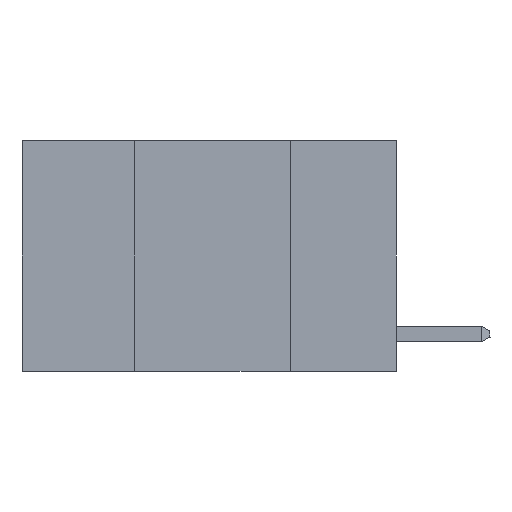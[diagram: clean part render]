
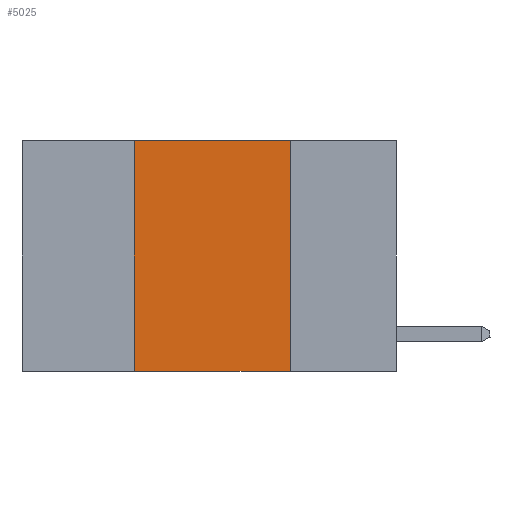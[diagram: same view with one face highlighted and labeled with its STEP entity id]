
A CAD part, left-side view. The second image highlights one B-rep face of the part: STEP entity #5025.
In plain terms, the highlighted planar face has unit normal (-1, 0, 0).
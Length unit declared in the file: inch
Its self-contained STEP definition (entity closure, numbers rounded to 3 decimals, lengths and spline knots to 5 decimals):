
#17 = LINE ( 'NONE', #2083, #7392 ) ;
#215 = CARTESIAN_POINT ( 'NONE',  ( 0., 0.42, 0. ) ) ;
#430 = CARTESIAN_POINT ( 'NONE',  ( 0., 0.6, 0. ) ) ;
#497 = EDGE_CURVE ( 'NONE', #7032, #1361, #4445, .T. ) ;
#557 = VERTEX_POINT ( 'NONE', #215 ) ;
#1181 = ORIENTED_EDGE ( 'NONE', *, *, #2107, .T. ) ;
#1361 = VERTEX_POINT ( 'NONE', #7373 ) ;
#1460 = CARTESIAN_POINT ( 'NONE',  ( 0., 0.17, 0. ) ) ;
#1609 = EDGE_CURVE ( 'NONE', #4319, #557, #2614, .T. ) ;
#1966 = DIRECTION ( 'NONE',  ( 0., 0., -1. ) ) ;
#1973 = DIRECTION ( 'NONE',  ( 0., -1., 0. ) ) ;
#2083 = CARTESIAN_POINT ( 'NONE',  ( 0., 0.6, -0.37 ) ) ;
#2107 = EDGE_CURVE ( 'NONE', #4319, #1361, #17, .T. ) ;
#2372 = ORIENTED_EDGE ( 'NONE', *, *, #1609, .F. ) ;
#2577 = PLANE ( 'NONE',  #3948 ) ;
#2614 = LINE ( 'NONE', #8236, #7128 ) ;
#3089 = ORIENTED_EDGE ( 'NONE', *, *, #4237, .F. ) ;
#3349 = CARTESIAN_POINT ( 'NONE',  ( 0., 0.6, 0. ) ) ;
#3557 = VECTOR ( 'NONE', #1973, 39.37008 ) ;
#3948 = AXIS2_PLACEMENT_3D ( 'NONE', #3349, #4789, #1966 ) ;
#4237 = EDGE_CURVE ( 'NONE', #557, #7032, #5991, .T. ) ;
#4319 = VERTEX_POINT ( 'NONE', #6318 ) ;
#4445 = LINE ( 'NONE', #8142, #8303 ) ;
#4789 = DIRECTION ( 'NONE',  ( 1., 0., 0. ) ) ;
#5025 = ADVANCED_FACE ( 'NONE', ( #6854 ), #2577, .F. ) ;
#5581 = ORIENTED_EDGE ( 'NONE', *, *, #497, .F. ) ;
#5991 = LINE ( 'NONE', #430, #3557 ) ;
#6318 = CARTESIAN_POINT ( 'NONE',  ( 0., 0.42, -0.37 ) ) ;
#6854 = FACE_OUTER_BOUND ( 'NONE', #7979, .T. ) ;
#7032 = VERTEX_POINT ( 'NONE', #1460 ) ;
#7128 = VECTOR ( 'NONE', #8287, 39.37008 ) ;
#7180 = DIRECTION ( 'NONE',  ( 0., 0., -1. ) ) ;
#7373 = CARTESIAN_POINT ( 'NONE',  ( 0., 0.17, -0.37 ) ) ;
#7392 = VECTOR ( 'NONE', #7786, 39.37008 ) ;
#7786 = DIRECTION ( 'NONE',  ( 0., -1., 0. ) ) ;
#7979 = EDGE_LOOP ( 'NONE', ( #5581, #3089, #2372, #1181 ) ) ;
#8142 = CARTESIAN_POINT ( 'NONE',  ( 0., 0.17, 0. ) ) ;
#8236 = CARTESIAN_POINT ( 'NONE',  ( 0., 0.42, 0. ) ) ;
#8287 = DIRECTION ( 'NONE',  ( 0., 0., 1. ) ) ;
#8303 = VECTOR ( 'NONE', #7180, 39.37008 ) ;
